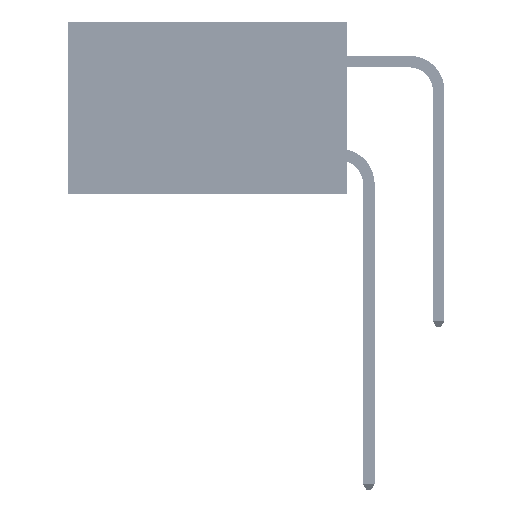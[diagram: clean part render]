
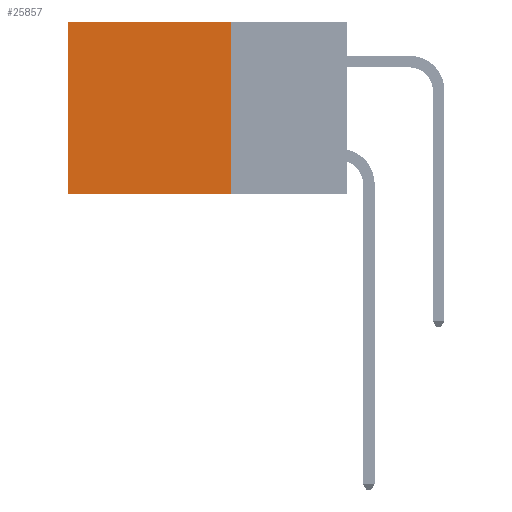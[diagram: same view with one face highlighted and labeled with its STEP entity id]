
A CAD part, left-side view. The second image highlights one B-rep face of the part: STEP entity #25857.
In plain terms, the highlighted planar face has unit normal (-1, 0, 0).
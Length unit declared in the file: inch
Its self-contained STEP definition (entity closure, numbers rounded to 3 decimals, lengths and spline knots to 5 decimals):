
#2608 = PLANE ( 'NONE',  #30070 ) ;
#2852 = ORIENTED_EDGE ( 'NONE', *, *, #44539, .F. ) ;
#4657 = ORIENTED_EDGE ( 'NONE', *, *, #40169, .T. ) ;
#5215 = VECTOR ( 'NONE', #21413, 39.37008 ) ;
#6724 = LINE ( 'NONE', #21879, #29128 ) ;
#7130 = EDGE_LOOP ( 'NONE', ( #4657, #2852, #20950, #30378 ) ) ;
#10457 = DIRECTION ( 'NONE',  ( 0., 0., -1. ) ) ;
#10497 = DIRECTION ( 'NONE',  ( 0., 0., -1. ) ) ;
#12280 = VERTEX_POINT ( 'NONE', #21989 ) ;
#18299 = CARTESIAN_POINT ( 'NONE',  ( 0.2875, 0.25, 0. ) ) ;
#18345 = CARTESIAN_POINT ( 'NONE',  ( 0.2875, 0.25, -0.37 ) ) ;
#18575 = DIRECTION ( 'NONE',  ( 0., 1., 0. ) ) ;
#20950 = ORIENTED_EDGE ( 'NONE', *, *, #30079, .F. ) ;
#21413 = DIRECTION ( 'NONE',  ( 0., 0., -1. ) ) ;
#21879 = CARTESIAN_POINT ( 'NONE',  ( 0.2875, 0.6, 0. ) ) ;
#21989 = CARTESIAN_POINT ( 'NONE',  ( 0.2875, 0.6, 0. ) ) ;
#25857 = ADVANCED_FACE ( 'NONE', ( #45396 ), #2608, .F. ) ;
#28785 = LINE ( 'NONE', #33564, #5215 ) ;
#29128 = VECTOR ( 'NONE', #10497, 39.37008 ) ;
#29306 = VECTOR ( 'NONE', #18575, 39.37008 ) ;
#30070 = AXIS2_PLACEMENT_3D ( 'NONE', #18299, #48936, #10457 ) ;
#30079 = EDGE_CURVE ( 'NONE', #37716, #43689, #28785, .T. ) ;
#30378 = ORIENTED_EDGE ( 'NONE', *, *, #39129, .T. ) ;
#33564 = CARTESIAN_POINT ( 'NONE',  ( 0.2875, 0.25, 0. ) ) ;
#37716 = VERTEX_POINT ( 'NONE', #44501 ) ;
#38969 = CARTESIAN_POINT ( 'NONE',  ( 0.2875, 0.6, -0.37 ) ) ;
#39129 = EDGE_CURVE ( 'NONE', #37716, #12280, #47433, .T. ) ;
#39570 = CARTESIAN_POINT ( 'NONE',  ( 0.2875, 0.25, 0. ) ) ;
#40169 = EDGE_CURVE ( 'NONE', #12280, #43838, #6724, .T. ) ;
#43689 = VERTEX_POINT ( 'NONE', #49090 ) ;
#43838 = VERTEX_POINT ( 'NONE', #38969 ) ;
#44126 = DIRECTION ( 'NONE',  ( 0., 1., 0. ) ) ;
#44501 = CARTESIAN_POINT ( 'NONE',  ( 0.2875, 0.25, 0. ) ) ;
#44539 = EDGE_CURVE ( 'NONE', #43689, #43838, #44955, .T. ) ;
#44955 = LINE ( 'NONE', #18345, #29306 ) ;
#45222 = VECTOR ( 'NONE', #44126, 39.37008 ) ;
#45396 = FACE_OUTER_BOUND ( 'NONE', #7130, .T. ) ;
#47433 = LINE ( 'NONE', #39570, #45222 ) ;
#48936 = DIRECTION ( 'NONE',  ( 1., 0., 0. ) ) ;
#49090 = CARTESIAN_POINT ( 'NONE',  ( 0.2875, 0.25, -0.37 ) ) ;
